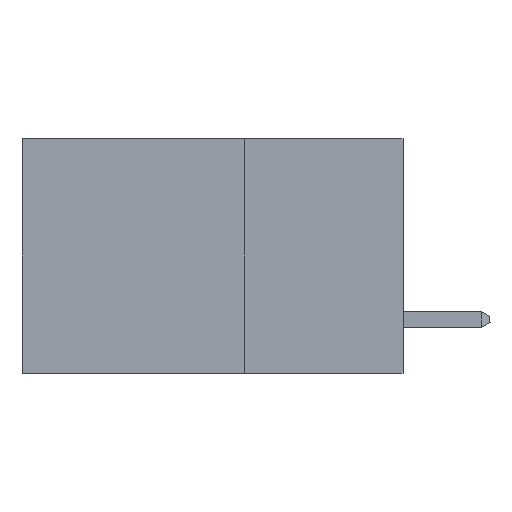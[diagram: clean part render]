
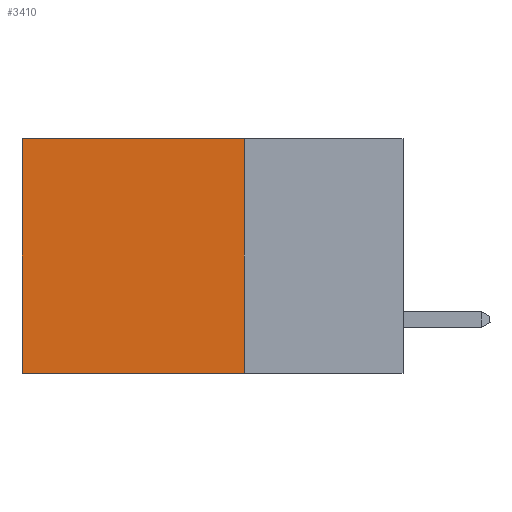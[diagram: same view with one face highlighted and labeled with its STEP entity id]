
A CAD part, left-side view. The second image highlights one B-rep face of the part: STEP entity #3410.
In plain terms, the highlighted planar face has unit normal (-1, 0, 0).
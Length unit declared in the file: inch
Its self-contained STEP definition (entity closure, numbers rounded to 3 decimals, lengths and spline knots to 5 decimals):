
#1 = LINE ( 'NONE', #7706, #5168 ) ;
#549 = LINE ( 'NONE', #9518, #6942 ) ;
#654 = DIRECTION ( 'NONE',  ( 0., 0., -1. ) ) ;
#771 = ORIENTED_EDGE ( 'NONE', *, *, #2326, .T. ) ;
#1226 = VECTOR ( 'NONE', #2888, 39.37008 ) ;
#2035 = ORIENTED_EDGE ( 'NONE', *, *, #2214, .F. ) ;
#2214 = EDGE_CURVE ( 'NONE', #6031, #7941, #1, .T. ) ;
#2326 = EDGE_CURVE ( 'NONE', #6031, #8653, #5696, .T. ) ;
#2888 = DIRECTION ( 'NONE',  ( 0., 1., 0. ) ) ;
#3323 = CARTESIAN_POINT ( 'NONE',  ( 0.2875, 0.25, 0. ) ) ;
#3410 = ADVANCED_FACE ( 'NONE', ( #4133 ), #8282, .F. ) ;
#3478 = CARTESIAN_POINT ( 'NONE',  ( 0.2875, 0.25, -0.37 ) ) ;
#3664 = CARTESIAN_POINT ( 'NONE',  ( 0.2875, 0.25, 0. ) ) ;
#3973 = VECTOR ( 'NONE', #4349, 39.37008 ) ;
#4133 = FACE_OUTER_BOUND ( 'NONE', #5868, .T. ) ;
#4166 = DIRECTION ( 'NONE',  ( 0., 0., -1. ) ) ;
#4199 = CARTESIAN_POINT ( 'NONE',  ( 0.2875, 0.6, -0.37 ) ) ;
#4349 = DIRECTION ( 'NONE',  ( 0., 1., 0. ) ) ;
#4653 = AXIS2_PLACEMENT_3D ( 'NONE', #3323, #7385, #4166 ) ;
#4918 = CARTESIAN_POINT ( 'NONE',  ( 0.2875, 0.25, 0. ) ) ;
#4935 = EDGE_CURVE ( 'NONE', #7941, #9402, #8355, .T. ) ;
#5168 = VECTOR ( 'NONE', #6908, 39.37008 ) ;
#5696 = LINE ( 'NONE', #3664, #1226 ) ;
#5697 = ORIENTED_EDGE ( 'NONE', *, *, #4935, .F. ) ;
#5797 = ORIENTED_EDGE ( 'NONE', *, *, #8604, .T. ) ;
#5868 = EDGE_LOOP ( 'NONE', ( #5797, #5697, #2035, #771 ) ) ;
#6031 = VERTEX_POINT ( 'NONE', #4918 ) ;
#6908 = DIRECTION ( 'NONE',  ( 0., 0., -1. ) ) ;
#6942 = VECTOR ( 'NONE', #654, 39.37008 ) ;
#7076 = CARTESIAN_POINT ( 'NONE',  ( 0.2875, 0.6, 0. ) ) ;
#7385 = DIRECTION ( 'NONE',  ( 1., 0., 0. ) ) ;
#7706 = CARTESIAN_POINT ( 'NONE',  ( 0.2875, 0.25, 0. ) ) ;
#7941 = VERTEX_POINT ( 'NONE', #3478 ) ;
#8282 = PLANE ( 'NONE',  #4653 ) ;
#8355 = LINE ( 'NONE', #9313, #3973 ) ;
#8604 = EDGE_CURVE ( 'NONE', #8653, #9402, #549, .T. ) ;
#8653 = VERTEX_POINT ( 'NONE', #7076 ) ;
#9313 = CARTESIAN_POINT ( 'NONE',  ( 0.2875, 0.25, -0.37 ) ) ;
#9402 = VERTEX_POINT ( 'NONE', #4199 ) ;
#9518 = CARTESIAN_POINT ( 'NONE',  ( 0.2875, 0.6, 0. ) ) ;
